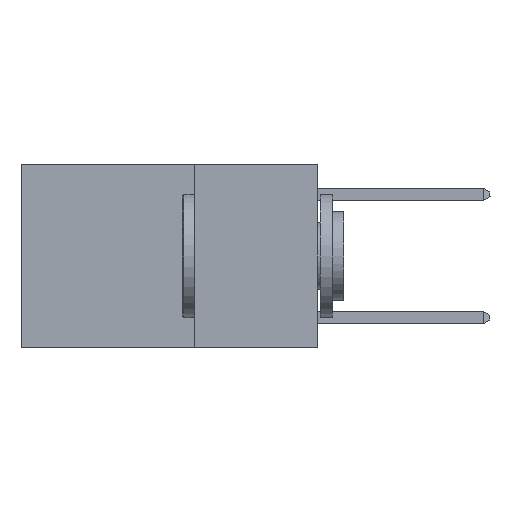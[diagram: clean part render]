
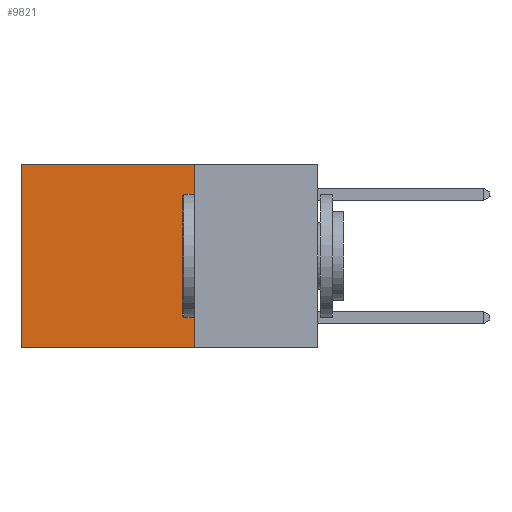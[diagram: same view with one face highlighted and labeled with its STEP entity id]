
A CAD part, left-side view. The second image highlights one B-rep face of the part: STEP entity #9821.
In plain terms, the highlighted planar face has unit normal (-1, 0, 0).
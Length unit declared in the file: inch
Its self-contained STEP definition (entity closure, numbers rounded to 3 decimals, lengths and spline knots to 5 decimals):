
#107 = CARTESIAN_POINT ( 'NONE',  ( 0.2625, 0.6, 0. ) ) ;
#177 = VERTEX_POINT ( 'NONE', #4526 ) ;
#332 = ORIENTED_EDGE ( 'NONE', *, *, #13853, .F. ) ;
#871 = CARTESIAN_POINT ( 'NONE',  ( 0.2625, 0.25, 0. ) ) ;
#1308 = CARTESIAN_POINT ( 'NONE',  ( 0.2625, 0.6, -0.37 ) ) ;
#1334 = DIRECTION ( 'NONE',  ( 0., 0., -1. ) ) ;
#2062 = PLANE ( 'NONE',  #11016 ) ;
#2160 = VECTOR ( 'NONE', #13294, 39.37008 ) ;
#2233 = DIRECTION ( 'NONE',  ( 0., 1., 0. ) ) ;
#2589 = VERTEX_POINT ( 'NONE', #1308 ) ;
#2666 = EDGE_LOOP ( 'NONE', ( #6008, #332, #12833, #13642 ) ) ;
#3116 = CARTESIAN_POINT ( 'NONE',  ( 0.2625, 0.25, 0. ) ) ;
#3903 = FACE_OUTER_BOUND ( 'NONE', #2666, .T. ) ;
#4526 = CARTESIAN_POINT ( 'NONE',  ( 0.2625, 0.25, 0. ) ) ;
#4913 = CARTESIAN_POINT ( 'NONE',  ( 0.2625, 0.25, -0.37 ) ) ;
#5236 = LINE ( 'NONE', #12556, #9170 ) ;
#5246 = EDGE_CURVE ( 'NONE', #177, #13436, #15358, .T. ) ;
#5334 = EDGE_CURVE ( 'NONE', #13436, #2589, #13466, .T. ) ;
#6008 = ORIENTED_EDGE ( 'NONE', *, *, #5334, .T. ) ;
#6318 = LINE ( 'NONE', #4913, #2160 ) ;
#7642 = VECTOR ( 'NONE', #2233, 39.37008 ) ;
#7761 = DIRECTION ( 'NONE',  ( 0., 0., -1. ) ) ;
#7826 = VECTOR ( 'NONE', #1334, 39.37008 ) ;
#9170 = VECTOR ( 'NONE', #7761, 39.37008 ) ;
#9548 = EDGE_CURVE ( 'NONE', #177, #14179, #5236, .T. ) ;
#9821 = ADVANCED_FACE ( 'NONE', ( #3903 ), #2062, .F. ) ;
#10848 = CARTESIAN_POINT ( 'NONE',  ( 0.2625, 0.25, -0.37 ) ) ;
#11016 = AXIS2_PLACEMENT_3D ( 'NONE', #3116, #11614, #11765 ) ;
#11614 = DIRECTION ( 'NONE',  ( 1., 0., 0. ) ) ;
#11765 = DIRECTION ( 'NONE',  ( 0., 0., -1. ) ) ;
#12556 = CARTESIAN_POINT ( 'NONE',  ( 0.2625, 0.25, 0. ) ) ;
#12833 = ORIENTED_EDGE ( 'NONE', *, *, #9548, .F. ) ;
#13294 = DIRECTION ( 'NONE',  ( 0., 1., 0. ) ) ;
#13436 = VERTEX_POINT ( 'NONE', #107 ) ;
#13466 = LINE ( 'NONE', #15586, #7826 ) ;
#13642 = ORIENTED_EDGE ( 'NONE', *, *, #5246, .T. ) ;
#13853 = EDGE_CURVE ( 'NONE', #14179, #2589, #6318, .T. ) ;
#14179 = VERTEX_POINT ( 'NONE', #10848 ) ;
#15358 = LINE ( 'NONE', #871, #7642 ) ;
#15586 = CARTESIAN_POINT ( 'NONE',  ( 0.2625, 0.6, 0. ) ) ;
